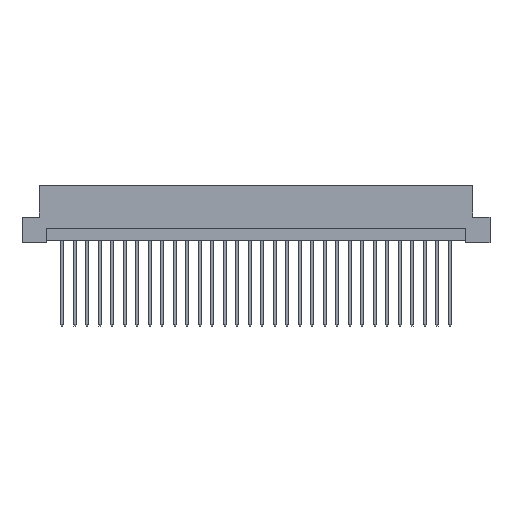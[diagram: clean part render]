
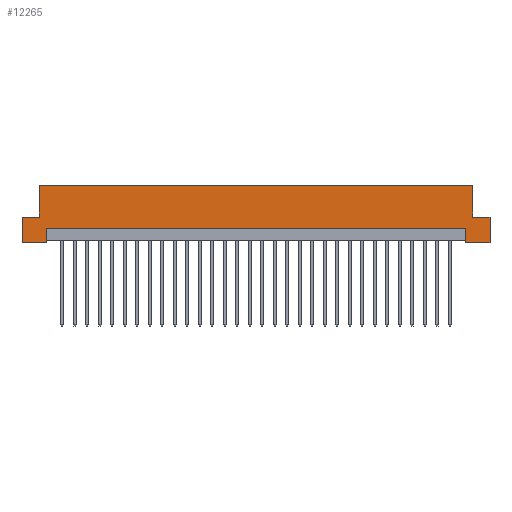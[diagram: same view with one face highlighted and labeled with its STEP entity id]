
A CAD part, front view. The second image highlights one B-rep face of the part: STEP entity #12265.
In plain terms, the highlighted planar face has unit normal (0, -1, 0).
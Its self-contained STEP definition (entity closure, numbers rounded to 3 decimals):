
#221 = EDGE_CURVE ( 'NONE', #2620, #14629, #6463, .T. ) ;
#253 = ORIENTED_EDGE ( 'NONE', *, *, #10661, .F. ) ;
#290 = VERTEX_POINT ( 'NONE', #10274 ) ;
#305 = CARTESIAN_POINT ( 'NONE',  ( 42.6, 0., 0.5 ) ) ;
#331 = EDGE_CURVE ( 'NONE', #13631, #4318, #10019, .T. ) ;
#362 = VECTOR ( 'NONE', #3247, 1000. ) ;
#444 = EDGE_CURVE ( 'NONE', #14629, #10765, #1567, .T. ) ;
#559 = VERTEX_POINT ( 'NONE', #4550 ) ;
#766 = ORIENTED_EDGE ( 'NONE', *, *, #221, .F. ) ;
#901 = CARTESIAN_POINT ( 'NONE',  ( -47.5, 0., 0. ) ) ;
#1019 = CARTESIAN_POINT ( 'NONE',  ( -47.5, 0., 5.2 ) ) ;
#1396 = CARTESIAN_POINT ( 'NONE',  ( -42.6, 0., 2.9 ) ) ;
#1567 = LINE ( 'NONE', #6546, #10176 ) ;
#1682 = CARTESIAN_POINT ( 'NONE',  ( -47.5, 0., 11.6 ) ) ;
#1696 = EDGE_LOOP ( 'NONE', ( #5234, #3370, #6564, #766, #4346, #6235, #14999, #14241, #253, #16026, #5391, #5826 ) ) ;
#2101 = CARTESIAN_POINT ( 'NONE',  ( 47.5, 0., 0. ) ) ;
#2620 = VERTEX_POINT ( 'NONE', #6869 ) ;
#2905 = VERTEX_POINT ( 'NONE', #6446 ) ;
#3095 = LINE ( 'NONE', #15610, #10058 ) ;
#3105 = LINE ( 'NONE', #13223, #10576 ) ;
#3247 = DIRECTION ( 'NONE',  ( 0., 0., 1. ) ) ;
#3262 = CARTESIAN_POINT ( 'NONE',  ( 44., 0., 5.2 ) ) ;
#3370 = ORIENTED_EDGE ( 'NONE', *, *, #10565, .T. ) ;
#3556 = CARTESIAN_POINT ( 'NONE',  ( -47.5, 0., 0. ) ) ;
#3682 = CARTESIAN_POINT ( 'NONE',  ( 42.6, 0., 0. ) ) ;
#4019 = VERTEX_POINT ( 'NONE', #1019 ) ;
#4188 = DIRECTION ( 'NONE',  ( 0., 0., -1. ) ) ;
#4318 = VERTEX_POINT ( 'NONE', #5096 ) ;
#4329 = DIRECTION ( 'NONE',  ( -1., 0., 0. ) ) ;
#4346 = ORIENTED_EDGE ( 'NONE', *, *, #13222, .F. ) ;
#4479 = CARTESIAN_POINT ( 'NONE',  ( 42.6, 0., 2.9 ) ) ;
#4550 = CARTESIAN_POINT ( 'NONE',  ( -44., 0., 11.6 ) ) ;
#4989 = VECTOR ( 'NONE', #15980, 1000. ) ;
#5096 = CARTESIAN_POINT ( 'NONE',  ( 44., 0., 11.6 ) ) ;
#5234 = ORIENTED_EDGE ( 'NONE', *, *, #14378, .F. ) ;
#5391 = ORIENTED_EDGE ( 'NONE', *, *, #11491, .F. ) ;
#5613 = VERTEX_POINT ( 'NONE', #4479 ) ;
#5698 = DIRECTION ( 'NONE',  ( 1., 0., 0. ) ) ;
#5826 = ORIENTED_EDGE ( 'NONE', *, *, #15744, .F. ) ;
#6182 = VECTOR ( 'NONE', #7547, 1000. ) ;
#6235 = ORIENTED_EDGE ( 'NONE', *, *, #331, .T. ) ;
#6357 = VECTOR ( 'NONE', #5698, 1000. ) ;
#6446 = CARTESIAN_POINT ( 'NONE',  ( -42.6, 0., 0. ) ) ;
#6463 = LINE ( 'NONE', #12597, #6182 ) ;
#6546 = CARTESIAN_POINT ( 'NONE',  ( -47.5, 0., 0. ) ) ;
#6564 = ORIENTED_EDGE ( 'NONE', *, *, #444, .F. ) ;
#6625 = DIRECTION ( 'NONE',  ( 0., 0., 1. ) ) ;
#6737 = DIRECTION ( 'NONE',  ( 0., 1., 0. ) ) ;
#6869 = CARTESIAN_POINT ( 'NONE',  ( 47.5, 0., 5.2 ) ) ;
#7170 = EDGE_CURVE ( 'NONE', #290, #559, #13277, .T. ) ;
#7542 = VECTOR ( 'NONE', #14606, 1000. ) ;
#7547 = DIRECTION ( 'NONE',  ( 0., 0., -1. ) ) ;
#8145 = PLANE ( 'NONE',  #15597 ) ;
#8166 = EDGE_CURVE ( 'NONE', #9316, #4019, #3105, .T. ) ;
#8224 = LINE ( 'NONE', #10547, #7542 ) ;
#8686 = LINE ( 'NONE', #901, #4989 ) ;
#8841 = VECTOR ( 'NONE', #6625, 1000. ) ;
#9300 = CARTESIAN_POINT ( 'NONE',  ( 42.6, 0., 2.9 ) ) ;
#9316 = VERTEX_POINT ( 'NONE', #3556 ) ;
#9393 = VERTEX_POINT ( 'NONE', #1396 ) ;
#10019 = LINE ( 'NONE', #15086, #8841 ) ;
#10058 = VECTOR ( 'NONE', #11870, 1000. ) ;
#10176 = VECTOR ( 'NONE', #11751, 1000. ) ;
#10274 = CARTESIAN_POINT ( 'NONE',  ( -44., 0., 5.2 ) ) ;
#10547 = CARTESIAN_POINT ( 'NONE',  ( -42.6, 0., 0.5 ) ) ;
#10565 = EDGE_CURVE ( 'NONE', #5613, #10765, #11649, .T. ) ;
#10576 = VECTOR ( 'NONE', #15951, 1000. ) ;
#10661 = EDGE_CURVE ( 'NONE', #4019, #290, #15801, .T. ) ;
#10765 = VERTEX_POINT ( 'NONE', #3682 ) ;
#10817 = DIRECTION ( 'NONE',  ( 1., 0., 0. ) ) ;
#11398 = VECTOR ( 'NONE', #4188, 1000. ) ;
#11491 = EDGE_CURVE ( 'NONE', #2905, #9316, #8686, .T. ) ;
#11632 = DIRECTION ( 'NONE',  ( 0., 0., 1. ) ) ;
#11649 = LINE ( 'NONE', #305, #11398 ) ;
#11694 = CARTESIAN_POINT ( 'NONE',  ( -44., 0., 5.2 ) ) ;
#11751 = DIRECTION ( 'NONE',  ( -1., 0., 0. ) ) ;
#11859 = LINE ( 'NONE', #9300, #15124 ) ;
#11870 = DIRECTION ( 'NONE',  ( 1., 0., 0. ) ) ;
#12265 = ADVANCED_FACE ( 'NONE', ( #13048 ), #8145, .F. ) ;
#12597 = CARTESIAN_POINT ( 'NONE',  ( 47.5, 0., 0. ) ) ;
#13048 = FACE_OUTER_BOUND ( 'NONE', #1696, .T. ) ;
#13222 = EDGE_CURVE ( 'NONE', #13631, #2620, #14490, .T. ) ;
#13223 = CARTESIAN_POINT ( 'NONE',  ( -47.5, 0., 0. ) ) ;
#13277 = LINE ( 'NONE', #11694, #362 ) ;
#13390 = CARTESIAN_POINT ( 'NONE',  ( -47.5, 0., 5.2 ) ) ;
#13414 = CARTESIAN_POINT ( 'NONE',  ( 47.5, 0., 5.2 ) ) ;
#13491 = EDGE_CURVE ( 'NONE', #559, #4318, #3095, .T. ) ;
#13631 = VERTEX_POINT ( 'NONE', #3262 ) ;
#14241 = ORIENTED_EDGE ( 'NONE', *, *, #7170, .F. ) ;
#14378 = EDGE_CURVE ( 'NONE', #5613, #9393, #11859, .T. ) ;
#14490 = LINE ( 'NONE', #13414, #6357 ) ;
#14606 = DIRECTION ( 'NONE',  ( 0., 0., -1. ) ) ;
#14629 = VERTEX_POINT ( 'NONE', #2101 ) ;
#14999 = ORIENTED_EDGE ( 'NONE', *, *, #13491, .F. ) ;
#15086 = CARTESIAN_POINT ( 'NONE',  ( 44., 0., 5.2 ) ) ;
#15124 = VECTOR ( 'NONE', #4329, 1000. ) ;
#15240 = VECTOR ( 'NONE', #10817, 1000. ) ;
#15597 = AXIS2_PLACEMENT_3D ( 'NONE', #1682, #6737, #11632 ) ;
#15610 = CARTESIAN_POINT ( 'NONE',  ( -47.5, 0., 11.6 ) ) ;
#15744 = EDGE_CURVE ( 'NONE', #9393, #2905, #8224, .T. ) ;
#15801 = LINE ( 'NONE', #13390, #15240 ) ;
#15951 = DIRECTION ( 'NONE',  ( 0., 0., 1. ) ) ;
#15980 = DIRECTION ( 'NONE',  ( -1., 0., 0. ) ) ;
#16026 = ORIENTED_EDGE ( 'NONE', *, *, #8166, .F. ) ;
